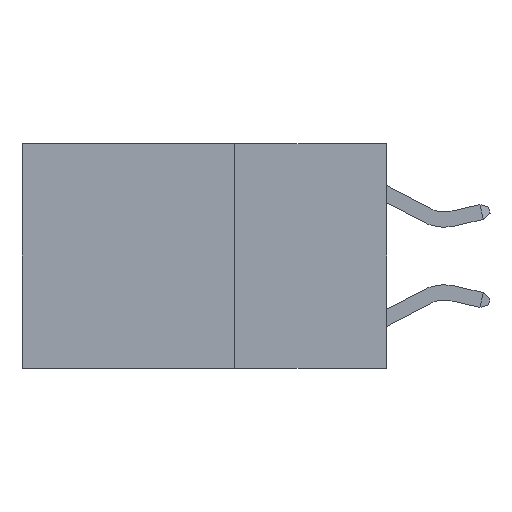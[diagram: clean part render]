
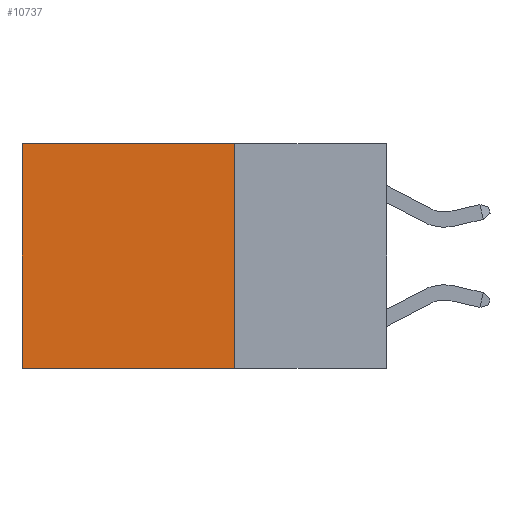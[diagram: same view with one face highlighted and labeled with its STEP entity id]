
A CAD part, left-side view. The second image highlights one B-rep face of the part: STEP entity #10737.
In plain terms, the highlighted planar face has unit normal (-1, 0, 0).
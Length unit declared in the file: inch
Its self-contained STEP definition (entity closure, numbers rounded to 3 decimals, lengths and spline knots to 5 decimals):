
#282 = ORIENTED_EDGE ( 'NONE', *, *, #5360, .F. ) ;
#308 = CARTESIAN_POINT ( 'NONE',  ( 0.2625, 0.25, 0. ) ) ;
#361 = DIRECTION ( 'NONE',  ( 1., 0., 0. ) ) ;
#498 = VECTOR ( 'NONE', #8934, 39.37008 ) ;
#691 = LINE ( 'NONE', #308, #3018 ) ;
#1707 = VERTEX_POINT ( 'NONE', #10014 ) ;
#2017 = EDGE_CURVE ( 'NONE', #2605, #1707, #10216, .T. ) ;
#2520 = DIRECTION ( 'NONE',  ( 0., 0., -1. ) ) ;
#2605 = VERTEX_POINT ( 'NONE', #6177 ) ;
#2990 = ORIENTED_EDGE ( 'NONE', *, *, #2017, .F. ) ;
#3018 = VECTOR ( 'NONE', #7431, 39.37008 ) ;
#3137 = LINE ( 'NONE', #12728, #498 ) ;
#4310 = CARTESIAN_POINT ( 'NONE',  ( 0.2625, 0.25, 0. ) ) ;
#5158 = VERTEX_POINT ( 'NONE', #5956 ) ;
#5160 = ORIENTED_EDGE ( 'NONE', *, *, #9560, .T. ) ;
#5358 = VECTOR ( 'NONE', #2520, 39.37008 ) ;
#5360 = EDGE_CURVE ( 'NONE', #7133, #2605, #3137, .T. ) ;
#5571 = EDGE_CURVE ( 'NONE', #5158, #1707, #7766, .T. ) ;
#5646 = AXIS2_PLACEMENT_3D ( 'NONE', #4310, #361, #7408 ) ;
#5877 = DIRECTION ( 'NONE',  ( 0., 1., 0. ) ) ;
#5956 = CARTESIAN_POINT ( 'NONE',  ( 0.2625, 0.6, 0. ) ) ;
#6177 = CARTESIAN_POINT ( 'NONE',  ( 0.2625, 0.25, -0.37 ) ) ;
#6379 = PLANE ( 'NONE',  #5646 ) ;
#7133 = VERTEX_POINT ( 'NONE', #10826 ) ;
#7408 = DIRECTION ( 'NONE',  ( 0., 0., -1. ) ) ;
#7431 = DIRECTION ( 'NONE',  ( 0., 1., 0. ) ) ;
#7706 = ORIENTED_EDGE ( 'NONE', *, *, #5571, .T. ) ;
#7766 = LINE ( 'NONE', #9525, #5358 ) ;
#7968 = VECTOR ( 'NONE', #5877, 39.37008 ) ;
#8369 = EDGE_LOOP ( 'NONE', ( #7706, #2990, #282, #5160 ) ) ;
#8934 = DIRECTION ( 'NONE',  ( 0., 0., -1. ) ) ;
#9122 = FACE_OUTER_BOUND ( 'NONE', #8369, .T. ) ;
#9525 = CARTESIAN_POINT ( 'NONE',  ( 0.2625, 0.6, 0. ) ) ;
#9560 = EDGE_CURVE ( 'NONE', #7133, #5158, #691, .T. ) ;
#10014 = CARTESIAN_POINT ( 'NONE',  ( 0.2625, 0.6, -0.37 ) ) ;
#10216 = LINE ( 'NONE', #11273, #7968 ) ;
#10737 = ADVANCED_FACE ( 'NONE', ( #9122 ), #6379, .F. ) ;
#10826 = CARTESIAN_POINT ( 'NONE',  ( 0.2625, 0.25, 0. ) ) ;
#11273 = CARTESIAN_POINT ( 'NONE',  ( 0.2625, 0.25, -0.37 ) ) ;
#12728 = CARTESIAN_POINT ( 'NONE',  ( 0.2625, 0.25, 0. ) ) ;
